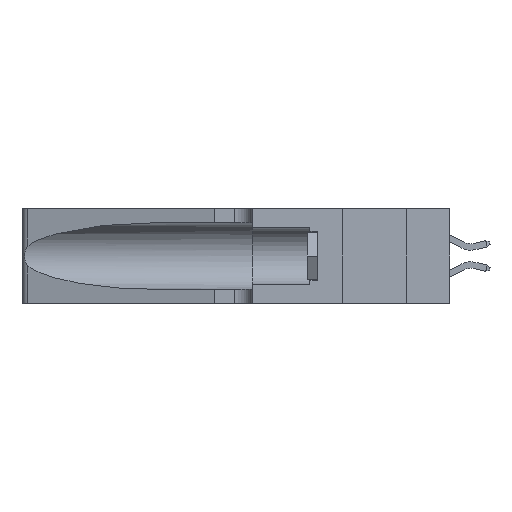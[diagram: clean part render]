
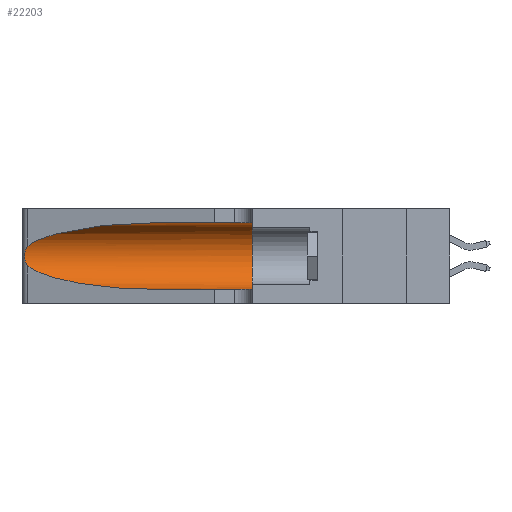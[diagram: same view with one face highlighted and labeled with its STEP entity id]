
A CAD part, left-side view. The second image highlights one B-rep face of the part: STEP entity #22203.
In plain terms, the highlighted cylindrical face has radius 3.308 mm (diameter 6.617 mm), a partial arc.
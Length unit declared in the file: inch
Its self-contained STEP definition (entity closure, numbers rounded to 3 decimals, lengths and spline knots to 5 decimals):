
#125 = ORIENTED_EDGE ( 'NONE', *, *, #14100, .T. ) ;
#341 = AXIS2_PLACEMENT_3D ( 'NONE', #8519, #17684, #26757 ) ;
#685 = EDGE_CURVE ( 'NONE', #4151, #13648, #8133, .T. ) ;
#1193 = CARTESIAN_POINT ( 'NONE',  ( 0.25789, 1.23486, 0.15765 ) ) ;
#2642 = CARTESIAN_POINT ( 'NONE',  ( 0.25487, 1.22718, 0.22369 ) ) ;
#2942 = CARTESIAN_POINT ( 'NONE',  ( 0.2373, 1.15595, 0.28018 ) ) ;
#3062 = VERTEX_POINT ( 'NONE', #3472 ) ;
#3461 = CARTESIAN_POINT ( 'NONE',  ( 0.25487, 1.22718, 0.22369 ) ) ;
#3472 = CARTESIAN_POINT ( 'NONE',  ( 0.1305, 0.35, 0.05475 ) ) ;
#4151 = VERTEX_POINT ( 'NONE', #14890 ) ;
#5336 = DIRECTION ( 'NONE',  ( 0., 0., -1. ) ) ;
#6655 = CARTESIAN_POINT ( 'NONE',  ( 0.25487, 1.22718, 0.14631 ) ) ;
#6757 = CARTESIAN_POINT ( 'NONE',  ( 0.1305, 1.61858, 0.05475 ) ) ;
#6834 = B_SPLINE_CURVE_WITH_KNOTS ( 'NONE', 3,
 ( #18727, #7865, #14643, #14944, #28382, #26305, #12548, #26411, #19535, #28279, #1193, #19228, #10174, #23951 ),
 .UNSPECIFIED., .F., .F.,
 ( 4, 2, 2, 2, 2, 2, 4 ),
 ( 0., 0.00027, 0.00053, 0.00107, 0.0016, 0.00187, 0.00214 ),
 .UNSPECIFIED. ) ;
#7295 = EDGE_CURVE ( 'NONE', #8705, #3062, #24114, .T. ) ;
#7382 = CARTESIAN_POINT ( 'NONE',  ( 0.18966, 0.96281, 0.31525 ) ) ;
#7845 = DIRECTION ( 'NONE',  ( 0., -1., 0. ) ) ;
#7865 = CARTESIAN_POINT ( 'NONE',  ( 0.25555, 1.22994, 0.2215 ) ) ;
#8133 =( BOUNDED_CURVE ( )  B_SPLINE_CURVE ( 3, ( #14072, #7382, #2942, #2642 ),
 .UNSPECIFIED., .F., .F. ) 
 B_SPLINE_CURVE_WITH_KNOTS ( ( 4, 4 ),
 ( 1.5708, 2.84003 ),
 .UNSPECIFIED. ) 
 CURVE ( )  GEOMETRIC_REPRESENTATION_ITEM ( )  RATIONAL_B_SPLINE_CURVE ( ( 1., 0.87, 0.87, 1. ) ) 
 REPRESENTATION_ITEM ( '' )  );
#8325 = LINE ( 'NONE', #27671, #28645 ) ;
#8519 = CARTESIAN_POINT ( 'NONE',  ( 0.1305, 0.35, 0.185 ) ) ;
#8705 = VERTEX_POINT ( 'NONE', #16041 ) ;
#8961 = CARTESIAN_POINT ( 'NONE',  ( 0.18966, 0.96281, 0.05475 ) ) ;
#9206 = AXIS2_PLACEMENT_3D ( 'NONE', #9658, #12214, #5336 ) ;
#9658 = CARTESIAN_POINT ( 'NONE',  ( 0.1305, 1.61858, 0.185 ) ) ;
#10051 = EDGE_CURVE ( 'NONE', #27639, #17106, #12692, .T. ) ;
#10174 = CARTESIAN_POINT ( 'NONE',  ( 0.25555, 1.22993, 0.14849 ) ) ;
#12214 = DIRECTION ( 'NONE',  ( 0., -1., 0. ) ) ;
#12548 = CARTESIAN_POINT ( 'NONE',  ( 0.26075, 1.23896, 0.19203 ) ) ;
#12615 = LINE ( 'NONE', #6757, #14037 ) ;
#12692 =( BOUNDED_CURVE ( )  B_SPLINE_CURVE ( 3, ( #6655, #25109, #8961, #13739 ),
 .UNSPECIFIED., .F., .F. ) 
 B_SPLINE_CURVE_WITH_KNOTS ( ( 4, 4 ),
 ( 3.44316, 4.71239 ),
 .UNSPECIFIED. ) 
 CURVE ( )  GEOMETRIC_REPRESENTATION_ITEM ( )  RATIONAL_B_SPLINE_CURVE ( ( 1., 0.87, 0.87, 1. ) ) 
 REPRESENTATION_ITEM ( '' )  );
#13062 = CYLINDRICAL_SURFACE ( 'NONE', #9206, 0.13025 ) ;
#13648 = VERTEX_POINT ( 'NONE', #3461 ) ;
#13739 = CARTESIAN_POINT ( 'NONE',  ( 0.1305, 0.72297, 0.05475 ) ) ;
#14037 = VECTOR ( 'NONE', #29596, 39.37008 ) ;
#14072 = CARTESIAN_POINT ( 'NONE',  ( 0.1305, 0.72297, 0.31525 ) ) ;
#14100 = EDGE_CURVE ( 'NONE', #13648, #27639, #6834, .T. ) ;
#14384 = ORIENTED_EDGE ( 'NONE', *, *, #7295, .F. ) ;
#14643 = CARTESIAN_POINT ( 'NONE',  ( 0.25639, 1.23184, 0.21858 ) ) ;
#14890 = CARTESIAN_POINT ( 'NONE',  ( 0.1305, 0.72297, 0.31525 ) ) ;
#14944 = CARTESIAN_POINT ( 'NONE',  ( 0.25787, 1.23484, 0.2124 ) ) ;
#16041 = CARTESIAN_POINT ( 'NONE',  ( 0.1305, 0.35, 0.31525 ) ) ;
#16612 = CARTESIAN_POINT ( 'NONE',  ( 0.25487, 1.22718, 0.14631 ) ) ;
#17106 = VERTEX_POINT ( 'NONE', #19050 ) ;
#17684 = DIRECTION ( 'NONE',  ( 0., 1., 0. ) ) ;
#18727 = CARTESIAN_POINT ( 'NONE',  ( 0.25487, 1.22718, 0.22369 ) ) ;
#19050 = CARTESIAN_POINT ( 'NONE',  ( 0.1305, 0.72297, 0.05475 ) ) ;
#19228 = CARTESIAN_POINT ( 'NONE',  ( 0.25639, 1.23186, 0.15144 ) ) ;
#19535 = CARTESIAN_POINT ( 'NONE',  ( 0.26017, 1.23833, 0.17102 ) ) ;
#20626 = ORIENTED_EDGE ( 'NONE', *, *, #23927, .T. ) ;
#22203 = ADVANCED_FACE ( 'NONE', ( #28344 ), #13062, .F. ) ;
#23927 = EDGE_CURVE ( 'NONE', #17106, #3062, #12615, .T. ) ;
#23951 = CARTESIAN_POINT ( 'NONE',  ( 0.25487, 1.22718, 0.14631 ) ) ;
#24107 = EDGE_CURVE ( 'NONE', #4151, #8705, #8325, .T. ) ;
#24114 = CIRCLE ( 'NONE', #341, 0.13025 ) ;
#25109 = CARTESIAN_POINT ( 'NONE',  ( 0.2373, 1.15595, 0.08982 ) ) ;
#26305 = CARTESIAN_POINT ( 'NONE',  ( 0.26018, 1.23835, 0.19895 ) ) ;
#26348 = ORIENTED_EDGE ( 'NONE', *, *, #10051, .T. ) ;
#26411 = CARTESIAN_POINT ( 'NONE',  ( 0.26075, 1.23896, 0.178 ) ) ;
#26757 = DIRECTION ( 'NONE',  ( 0., 0., 1. ) ) ;
#26940 = ORIENTED_EDGE ( 'NONE', *, *, #685, .T. ) ;
#27387 = ORIENTED_EDGE ( 'NONE', *, *, #24107, .F. ) ;
#27639 = VERTEX_POINT ( 'NONE', #16612 ) ;
#27671 = CARTESIAN_POINT ( 'NONE',  ( 0.1305, 1.61858, 0.31525 ) ) ;
#27819 = EDGE_LOOP ( 'NONE', ( #26940, #125, #26348, #20626, #14384, #27387 ) ) ;
#28279 = CARTESIAN_POINT ( 'NONE',  ( 0.25856, 1.23593, 0.16098 ) ) ;
#28344 = FACE_OUTER_BOUND ( 'NONE', #27819, .T. ) ;
#28382 = CARTESIAN_POINT ( 'NONE',  ( 0.25854, 1.2359, 0.20912 ) ) ;
#28645 = VECTOR ( 'NONE', #7845, 39.37008 ) ;
#29596 = DIRECTION ( 'NONE',  ( 0., -1., 0. ) ) ;
